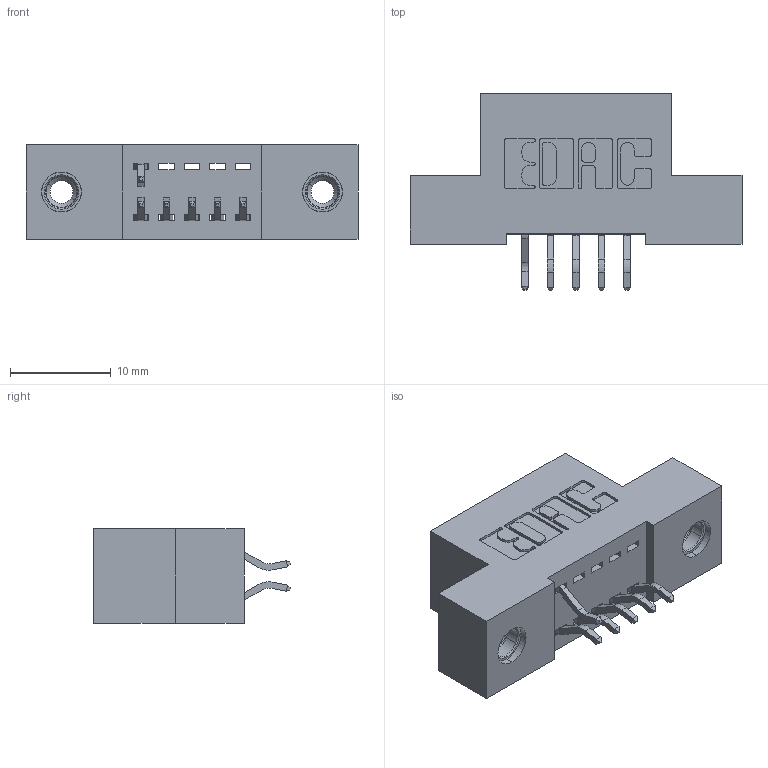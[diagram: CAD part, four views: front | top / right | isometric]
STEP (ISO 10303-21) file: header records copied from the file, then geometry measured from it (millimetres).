
FILE_DESCRIPTION (( 'STEP AP203' ), '1' );
FILE_NAME ('342-010-556-208.STEP', '2018-08-10T13:57:44', ( '' ), ( '' ), 'SwSTEP 2.0', 'SolidWorks 2016', '' );
FILE_SCHEMA (( 'CONFIG_CONTROL_DESIGN' ));
Length unit declared in the file: inch
Products named in the file (4): 342 Part_TI; 345-292-001_556 Tail; 345-250-001_345-250-003-102; 342-010-556-208
Assembly tree (9 placements, depth 2):
  342-010-556-208
    342 Part_TI
    345-292-001_556 Tail  x6
    345-250-001_345-250-003-102  x2
Bounding box: 33.02 x 19.58 x 9.4 mm (x, y, z)
Volume: 2749.9 mm3; surface area: 3369.9 mm2
Topology: 9 solids, 9 shells, 542 faces, 1557 edges, 1022 vertices
Faces by surface type: plane 362, cylinder 164, cone 12, torus 4
Entity records: 9148 total; most frequent: CARTESIAN_POINT 1573, ORIENTED_EDGE 1494, DIRECTION 1425, EDGE_CURVE 747, VECTOR 591, LINE 591, VERTEX_POINT 492, AXIS2_PLACEMENT_3D 417
